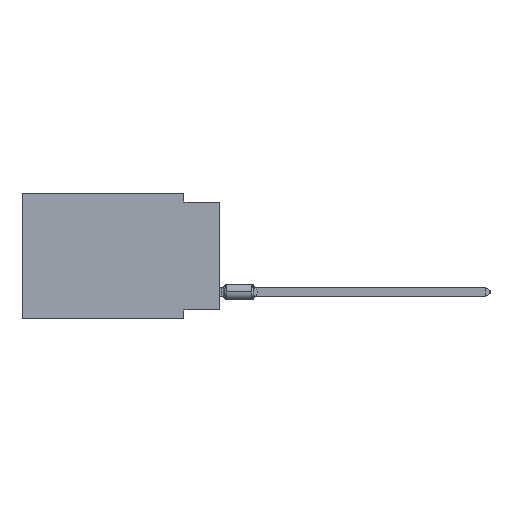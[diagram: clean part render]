
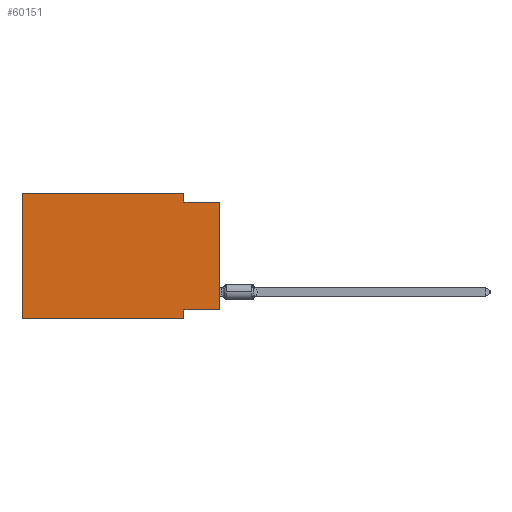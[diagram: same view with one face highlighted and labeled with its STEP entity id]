
A CAD part, left-side view. The second image highlights one B-rep face of the part: STEP entity #60151.
In plain terms, the highlighted planar face has unit normal (-1, 0, 0).
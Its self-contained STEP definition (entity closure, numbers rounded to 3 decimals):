
#451 = CARTESIAN_POINT ( 'NONE',  ( 0., 0., -0.635 ) ) ;
#1063 = LINE ( 'NONE', #451, #35229 ) ;
#1929 = CARTESIAN_POINT ( 'NONE',  ( 0., 13.97, 0. ) ) ;
#3558 = EDGE_CURVE ( 'NONE', #12938, #55812, #26453, .T. ) ;
#4873 = ORIENTED_EDGE ( 'NONE', *, *, #3558, .F. ) ;
#5295 = EDGE_LOOP ( 'NONE', ( #32359, #60591, #4873, #43653, #22874, #49571, #34978, #6544 ) ) ;
#6348 = EDGE_CURVE ( 'NONE', #31518, #18531, #29916, .T. ) ;
#6544 = ORIENTED_EDGE ( 'NONE', *, *, #6348, .F. ) ;
#7738 = VECTOR ( 'NONE', #52909, 1000. ) ;
#11827 = CARTESIAN_POINT ( 'NONE',  ( 0., 2.54, -8.89 ) ) ;
#12068 = VERTEX_POINT ( 'NONE', #45314 ) ;
#12938 = VERTEX_POINT ( 'NONE', #37380 ) ;
#14445 = CARTESIAN_POINT ( 'NONE',  ( 0., 13.97, 0. ) ) ;
#14713 = VECTOR ( 'NONE', #43095, 1000. ) ;
#15410 = DIRECTION ( 'NONE',  ( 0., -1., 0. ) ) ;
#15933 = VECTOR ( 'NONE', #42389, 1000. ) ;
#16356 = VECTOR ( 'NONE', #45802, 1000. ) ;
#18531 = VERTEX_POINT ( 'NONE', #29722 ) ;
#19930 = EDGE_CURVE ( 'NONE', #18531, #48958, #38850, .T. ) ;
#20277 = CARTESIAN_POINT ( 'NONE',  ( 0., 13.97, 0. ) ) ;
#20433 = CARTESIAN_POINT ( 'NONE',  ( 0., 2.54, -8.89 ) ) ;
#22874 = ORIENTED_EDGE ( 'NONE', *, *, #50903, .F. ) ;
#23558 = CARTESIAN_POINT ( 'NONE',  ( 0., 0., -8.255 ) ) ;
#23822 = CARTESIAN_POINT ( 'NONE',  ( 0., 13.97, 0. ) ) ;
#25225 = VECTOR ( 'NONE', #15410, 1000. ) ;
#26191 = VERTEX_POINT ( 'NONE', #1929 ) ;
#26453 = LINE ( 'NONE', #40801, #16356 ) ;
#26911 = CARTESIAN_POINT ( 'NONE',  ( 0., 2.54, -0.635 ) ) ;
#28482 = DIRECTION ( 'NONE',  ( 1., 0., 0. ) ) ;
#28739 = VECTOR ( 'NONE', #57246, 1000. ) ;
#29083 = EDGE_CURVE ( 'NONE', #31518, #12068, #46449, .T. ) ;
#29401 = VECTOR ( 'NONE', #54263, 1000. ) ;
#29722 = CARTESIAN_POINT ( 'NONE',  ( 0., 2.54, -8.255 ) ) ;
#29916 = LINE ( 'NONE', #40203, #29401 ) ;
#31518 = VERTEX_POINT ( 'NONE', #23558 ) ;
#32359 = ORIENTED_EDGE ( 'NONE', *, *, #29083, .T. ) ;
#34445 = LINE ( 'NONE', #43829, #25225 ) ;
#34978 = ORIENTED_EDGE ( 'NONE', *, *, #19930, .F. ) ;
#35229 = VECTOR ( 'NONE', #56967, 1000. ) ;
#37380 = CARTESIAN_POINT ( 'NONE',  ( 0., 2.54, 0. ) ) ;
#37842 = FACE_OUTER_BOUND ( 'NONE', #5295, .T. ) ;
#38770 = DIRECTION ( 'NONE',  ( 0., 0., -1. ) ) ;
#38850 = LINE ( 'NONE', #20433, #7738 ) ;
#40194 = AXIS2_PLACEMENT_3D ( 'NONE', #14445, #28482, #38770 ) ;
#40203 = CARTESIAN_POINT ( 'NONE',  ( 0., 0., -8.255 ) ) ;
#40801 = CARTESIAN_POINT ( 'NONE',  ( 0., 2.54, 0. ) ) ;
#42208 = EDGE_CURVE ( 'NONE', #52053, #48958, #34445, .T. ) ;
#42389 = DIRECTION ( 'NONE',  ( 0., 0., 1. ) ) ;
#42849 = PLANE ( 'NONE',  #40194 ) ;
#43095 = DIRECTION ( 'NONE',  ( 0., -1., 0. ) ) ;
#43653 = ORIENTED_EDGE ( 'NONE', *, *, #48870, .F. ) ;
#43829 = CARTESIAN_POINT ( 'NONE',  ( 0., 13.97, -8.89 ) ) ;
#45314 = CARTESIAN_POINT ( 'NONE',  ( 0., 0., -0.635 ) ) ;
#45802 = DIRECTION ( 'NONE',  ( 0., 0., -1. ) ) ;
#46449 = LINE ( 'NONE', #55801, #15933 ) ;
#47569 = LINE ( 'NONE', #23822, #28739 ) ;
#48870 = EDGE_CURVE ( 'NONE', #26191, #12938, #57453, .T. ) ;
#48958 = VERTEX_POINT ( 'NONE', #11827 ) ;
#49571 = ORIENTED_EDGE ( 'NONE', *, *, #42208, .T. ) ;
#50903 = EDGE_CURVE ( 'NONE', #52053, #26191, #47569, .T. ) ;
#52053 = VERTEX_POINT ( 'NONE', #57990 ) ;
#52909 = DIRECTION ( 'NONE',  ( 0., 0., -1. ) ) ;
#54263 = DIRECTION ( 'NONE',  ( 0., 1., 0. ) ) ;
#55801 = CARTESIAN_POINT ( 'NONE',  ( 0., 0., 0. ) ) ;
#55812 = VERTEX_POINT ( 'NONE', #26911 ) ;
#56723 = EDGE_CURVE ( 'NONE', #55812, #12068, #1063, .T. ) ;
#56967 = DIRECTION ( 'NONE',  ( 0., -1., 0. ) ) ;
#57246 = DIRECTION ( 'NONE',  ( 0., 0., 1. ) ) ;
#57453 = LINE ( 'NONE', #20277, #14713 ) ;
#57990 = CARTESIAN_POINT ( 'NONE',  ( 0., 13.97, -8.89 ) ) ;
#60151 = ADVANCED_FACE ( 'NONE', ( #37842 ), #42849, .F. ) ;
#60591 = ORIENTED_EDGE ( 'NONE', *, *, #56723, .F. ) ;
